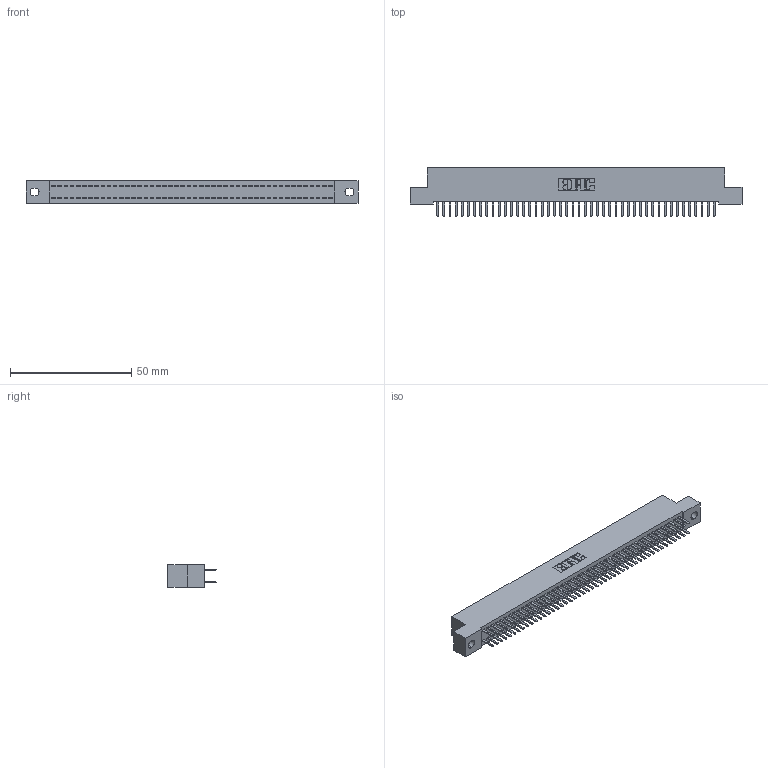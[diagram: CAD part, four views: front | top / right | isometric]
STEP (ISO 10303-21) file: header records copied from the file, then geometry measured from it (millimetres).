
FILE_DESCRIPTION (( 'STEP AP203' ), '1' );
FILE_NAME ('392-092-520-202.STEP', '2018-08-18T07:36:34', ( '' ), ( '' ), 'SwSTEP 2.0', 'SolidWorks 2016', '' );
FILE_SCHEMA (( 'CONFIG_CONTROL_DESIGN' ));
Length unit declared in the file: inch
Products named in the file (3): 342 Part_.128 Slot; 345-292-001_345-293-120; 392-092-520-202
Assembly tree (93 placements, depth 2):
  392-092-520-202
    342 Part_.128 Slot
    345-292-001_345-293-120  x92
Bounding box: 137.16 x 20.02 x 9.4 mm (x, y, z)
Volume: 12250.1 mm3; surface area: 19702.8 mm2
Topology: 93 solids, 93 shells, 5266 faces, 15307 edges, 9958 vertices
Faces by surface type: plane 3566, cylinder 1700
Entity records: 29193 total; most frequent: CARTESIAN_POINT 4846, ORIENTED_EDGE 4770, DIRECTION 4121, EDGE_CURVE 2385, VECTOR 2253, LINE 2253, VERTEX_POINT 1586, AXIS2_PLACEMENT_3D 934
